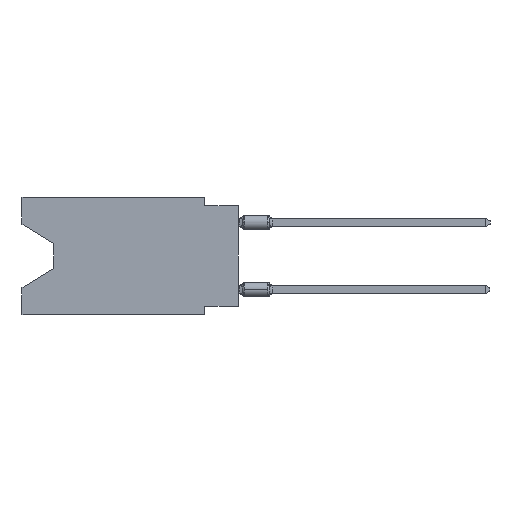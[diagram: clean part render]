
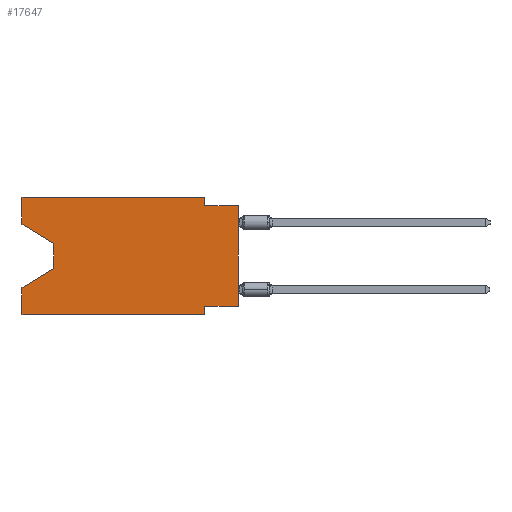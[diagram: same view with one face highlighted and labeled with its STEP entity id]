
A CAD part, left-side view. The second image highlights one B-rep face of the part: STEP entity #17647.
In plain terms, the highlighted planar face has unit normal (-1, 0, 0).
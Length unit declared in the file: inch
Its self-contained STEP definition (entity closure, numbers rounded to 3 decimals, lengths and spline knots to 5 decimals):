
#181 = CARTESIAN_POINT ( 'NONE',  ( 0., 0.55, -0.138 ) ) ;
#519 = LINE ( 'NONE', #10033, #2026 ) ;
#553 = CARTESIAN_POINT ( 'NONE',  ( 0., 0.645, -0.35 ) ) ;
#668 = ORIENTED_EDGE ( 'NONE', *, *, #9347, .F. ) ;
#994 = CARTESIAN_POINT ( 'NONE',  ( 0., 0.645, -0.08025 ) ) ;
#1235 = ORIENTED_EDGE ( 'NONE', *, *, #4958, .T. ) ;
#1237 = VECTOR ( 'NONE', #7098, 39.37008 ) ;
#1342 = LINE ( 'NONE', #17765, #14577 ) ;
#1566 = DIRECTION ( 'NONE',  ( 0., -1., 0. ) ) ;
#1686 = CARTESIAN_POINT ( 'NONE',  ( 0., 0., -0.325 ) ) ;
#1836 = LINE ( 'NONE', #4626, #5623 ) ;
#2026 = VECTOR ( 'NONE', #17010, 39.37008 ) ;
#2087 = CARTESIAN_POINT ( 'NONE',  ( 0., 0.1, -0.35 ) ) ;
#2415 = EDGE_CURVE ( 'NONE', #7218, #18115, #12493, .T. ) ;
#2442 = VERTEX_POINT ( 'NONE', #12670 ) ;
#2976 = CARTESIAN_POINT ( 'NONE',  ( 0., 0.645, 0. ) ) ;
#3080 = VERTEX_POINT ( 'NONE', #553 ) ;
#3097 = VERTEX_POINT ( 'NONE', #14692 ) ;
#3419 = VECTOR ( 'NONE', #13824, 39.37008 ) ;
#3442 = PLANE ( 'NONE',  #7649 ) ;
#3580 = CARTESIAN_POINT ( 'NONE',  ( 0., 0.645, 0. ) ) ;
#3824 = VECTOR ( 'NONE', #1566, 39.37008 ) ;
#4057 = VECTOR ( 'NONE', #8670, 39.37008 ) ;
#4209 = CARTESIAN_POINT ( 'NONE',  ( 0., 0., -0.025 ) ) ;
#4257 = EDGE_CURVE ( 'NONE', #15754, #11556, #14441, .T. ) ;
#4548 = CARTESIAN_POINT ( 'NONE',  ( 0., 0., -0.025 ) ) ;
#4626 = CARTESIAN_POINT ( 'NONE',  ( 0., 0.645, -0.35 ) ) ;
#4716 = EDGE_CURVE ( 'NONE', #11556, #12564, #519, .T. ) ;
#4958 = EDGE_CURVE ( 'NONE', #15754, #12650, #9613, .T. ) ;
#5336 = DIRECTION ( 'NONE',  ( 0., -1., 0. ) ) ;
#5339 = ORIENTED_EDGE ( 'NONE', *, *, #4257, .F. ) ;
#5623 = VECTOR ( 'NONE', #15976, 39.37008 ) ;
#6110 = LINE ( 'NONE', #3580, #17093 ) ;
#6138 = CARTESIAN_POINT ( 'NONE',  ( 0., 0.55, -0.212 ) ) ;
#6294 = DIRECTION ( 'NONE',  ( 0., 0., 1. ) ) ;
#7000 = LINE ( 'NONE', #4209, #9387 ) ;
#7098 = DIRECTION ( 'NONE',  ( 0., 0., -1. ) ) ;
#7115 = VECTOR ( 'NONE', #14569, 39.37008 ) ;
#7218 = VERTEX_POINT ( 'NONE', #181 ) ;
#7429 = EDGE_CURVE ( 'NONE', #11367, #7218, #12447, .T. ) ;
#7649 = AXIS2_PLACEMENT_3D ( 'NONE', #8942, #13054, #14624 ) ;
#8282 = ORIENTED_EDGE ( 'NONE', *, *, #8679, .T. ) ;
#8607 = DIRECTION ( 'NONE',  ( 0., 0., 1. ) ) ;
#8663 = CARTESIAN_POINT ( 'NONE',  ( 0., 0.645, 0. ) ) ;
#8670 = DIRECTION ( 'NONE',  ( 0., 1., 0. ) ) ;
#8679 = EDGE_CURVE ( 'NONE', #18115, #2442, #11121, .T. ) ;
#8908 = EDGE_CURVE ( 'NONE', #3080, #2442, #6110, .T. ) ;
#8942 = CARTESIAN_POINT ( 'NONE',  ( 0., 0.645, 0. ) ) ;
#9347 = EDGE_CURVE ( 'NONE', #16309, #12650, #7000, .T. ) ;
#9387 = VECTOR ( 'NONE', #5336, 39.37008 ) ;
#9613 = LINE ( 'NONE', #15664, #16008 ) ;
#9807 = EDGE_CURVE ( 'NONE', #3080, #12564, #1836, .T. ) ;
#10033 = CARTESIAN_POINT ( 'NONE',  ( 0., 0.1, -0.35 ) ) ;
#10129 = LINE ( 'NONE', #2976, #3824 ) ;
#10185 = LINE ( 'NONE', #17349, #7115 ) ;
#10220 = EDGE_CURVE ( 'NONE', #3097, #16309, #10185, .T. ) ;
#10260 = ORIENTED_EDGE ( 'NONE', *, *, #7429, .T. ) ;
#10589 = DIRECTION ( 'NONE',  ( 0., 0., 1. ) ) ;
#11121 = LINE ( 'NONE', #15401, #3419 ) ;
#11367 = VERTEX_POINT ( 'NONE', #12978 ) ;
#11415 = CARTESIAN_POINT ( 'NONE',  ( 0., 0.1, -0.325 ) ) ;
#11543 = EDGE_LOOP ( 'NONE', ( #10260, #14308, #8282, #14557, #16931, #12733, #5339, #1235, #668, #17613, #17888, #18328 ) ) ;
#11556 = VERTEX_POINT ( 'NONE', #11415 ) ;
#11914 = CARTESIAN_POINT ( 'NONE',  ( 0., 0., -0.325 ) ) ;
#12447 = LINE ( 'NONE', #994, #14097 ) ;
#12493 = LINE ( 'NONE', #18347, #1237 ) ;
#12564 = VERTEX_POINT ( 'NONE', #2087 ) ;
#12650 = VERTEX_POINT ( 'NONE', #4548 ) ;
#12670 = CARTESIAN_POINT ( 'NONE',  ( 0., 0.645, -0.26975 ) ) ;
#12733 = ORIENTED_EDGE ( 'NONE', *, *, #4716, .F. ) ;
#12743 = EDGE_CURVE ( 'NONE', #14946, #3097, #10129, .T. ) ;
#12978 = CARTESIAN_POINT ( 'NONE',  ( 0., 0.645, -0.08025 ) ) ;
#13054 = DIRECTION ( 'NONE',  ( 1., 0., 0. ) ) ;
#13137 = FACE_OUTER_BOUND ( 'NONE', #11543, .T. ) ;
#13824 = DIRECTION ( 'NONE',  ( 0., 0.855, -0.519 ) ) ;
#14097 = VECTOR ( 'NONE', #15229, 39.37008 ) ;
#14308 = ORIENTED_EDGE ( 'NONE', *, *, #2415, .T. ) ;
#14441 = LINE ( 'NONE', #1686, #4057 ) ;
#14557 = ORIENTED_EDGE ( 'NONE', *, *, #8908, .F. ) ;
#14569 = DIRECTION ( 'NONE',  ( 0., 0., -1. ) ) ;
#14577 = VECTOR ( 'NONE', #10589, 39.37008 ) ;
#14624 = DIRECTION ( 'NONE',  ( 0., 0., -1. ) ) ;
#14692 = CARTESIAN_POINT ( 'NONE',  ( 0., 0.1, 0. ) ) ;
#14946 = VERTEX_POINT ( 'NONE', #8663 ) ;
#15229 = DIRECTION ( 'NONE',  ( 0., -0.855, -0.519 ) ) ;
#15401 = CARTESIAN_POINT ( 'NONE',  ( 0., 0.55, -0.212 ) ) ;
#15664 = CARTESIAN_POINT ( 'NONE',  ( 0., 0., 0. ) ) ;
#15754 = VERTEX_POINT ( 'NONE', #11914 ) ;
#15839 = EDGE_CURVE ( 'NONE', #11367, #14946, #1342, .T. ) ;
#15976 = DIRECTION ( 'NONE',  ( 0., -1., 0. ) ) ;
#16008 = VECTOR ( 'NONE', #8607, 39.37008 ) ;
#16309 = VERTEX_POINT ( 'NONE', #18085 ) ;
#16931 = ORIENTED_EDGE ( 'NONE', *, *, #9807, .T. ) ;
#17010 = DIRECTION ( 'NONE',  ( 0., 0., -1. ) ) ;
#17093 = VECTOR ( 'NONE', #6294, 39.37008 ) ;
#17349 = CARTESIAN_POINT ( 'NONE',  ( 0., 0.1, 0. ) ) ;
#17613 = ORIENTED_EDGE ( 'NONE', *, *, #10220, .F. ) ;
#17647 = ADVANCED_FACE ( 'NONE', ( #13137 ), #3442, .F. ) ;
#17765 = CARTESIAN_POINT ( 'NONE',  ( 0., 0.645, 0. ) ) ;
#17888 = ORIENTED_EDGE ( 'NONE', *, *, #12743, .F. ) ;
#18085 = CARTESIAN_POINT ( 'NONE',  ( 0., 0.1, -0.025 ) ) ;
#18115 = VERTEX_POINT ( 'NONE', #6138 ) ;
#18328 = ORIENTED_EDGE ( 'NONE', *, *, #15839, .F. ) ;
#18347 = CARTESIAN_POINT ( 'NONE',  ( 0., 0.55, -0.138 ) ) ;
